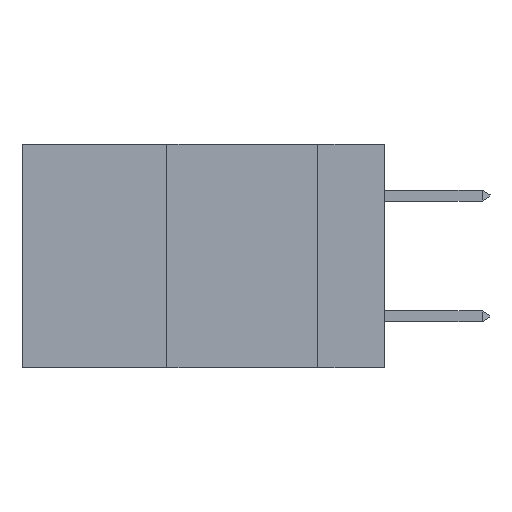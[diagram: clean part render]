
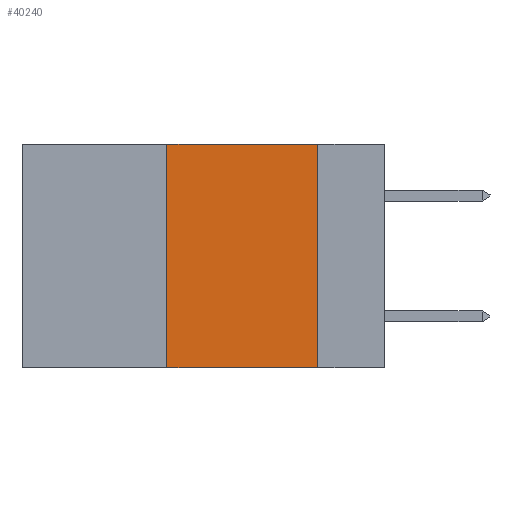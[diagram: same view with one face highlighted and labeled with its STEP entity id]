
A CAD part, left-side view. The second image highlights one B-rep face of the part: STEP entity #40240.
In plain terms, the highlighted planar face has unit normal (-1, 0, 0).
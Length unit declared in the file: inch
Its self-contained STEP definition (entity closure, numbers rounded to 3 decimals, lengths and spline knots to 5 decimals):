
#929 = ORIENTED_EDGE ( 'NONE', *, *, #5429, .F. ) ;
#1715 = EDGE_CURVE ( 'NONE', #12035, #21462, #6893, .T. ) ;
#3799 = EDGE_LOOP ( 'NONE', ( #34235, #929, #30541, #20647 ) ) ;
#4870 = FACE_OUTER_BOUND ( 'NONE', #3799, .T. ) ;
#5429 = EDGE_CURVE ( 'NONE', #21462, #37367, #34326, .T. ) ;
#5641 = EDGE_CURVE ( 'NONE', #12035, #15205, #41756, .T. ) ;
#5966 = CARTESIAN_POINT ( 'NONE',  ( 0., 0.11, 0. ) ) ;
#6170 = CARTESIAN_POINT ( 'NONE',  ( 0., 0.6, -0.37 ) ) ;
#6893 = LINE ( 'NONE', #16922, #13114 ) ;
#11498 = DIRECTION ( 'NONE',  ( 0., 0., -1. ) ) ;
#12035 = VERTEX_POINT ( 'NONE', #40490 ) ;
#12129 = EDGE_CURVE ( 'NONE', #37367, #15205, #12585, .T. ) ;
#12585 = LINE ( 'NONE', #5966, #29763 ) ;
#13114 = VECTOR ( 'NONE', #32696, 39.37008 ) ;
#15205 = VERTEX_POINT ( 'NONE', #28872 ) ;
#16389 = CARTESIAN_POINT ( 'NONE',  ( 0., 0.36, 0. ) ) ;
#16922 = CARTESIAN_POINT ( 'NONE',  ( 0., 0.36, 0. ) ) ;
#20647 = ORIENTED_EDGE ( 'NONE', *, *, #5641, .T. ) ;
#21462 = VERTEX_POINT ( 'NONE', #16389 ) ;
#21908 = AXIS2_PLACEMENT_3D ( 'NONE', #31096, #28131, #11498 ) ;
#21956 = DIRECTION ( 'NONE',  ( 0., -1., 0. ) ) ;
#22389 = VECTOR ( 'NONE', #21956, 39.37008 ) ;
#27395 = CARTESIAN_POINT ( 'NONE',  ( 0., 0.11, 0. ) ) ;
#27505 = DIRECTION ( 'NONE',  ( 0., -1., 0. ) ) ;
#28131 = DIRECTION ( 'NONE',  ( 1., 0., 0. ) ) ;
#28872 = CARTESIAN_POINT ( 'NONE',  ( 0., 0.11, -0.37 ) ) ;
#29763 = VECTOR ( 'NONE', #31982, 39.37008 ) ;
#29866 = VECTOR ( 'NONE', #27505, 39.37008 ) ;
#30541 = ORIENTED_EDGE ( 'NONE', *, *, #1715, .F. ) ;
#31096 = CARTESIAN_POINT ( 'NONE',  ( 0., 0.6, 0. ) ) ;
#31982 = DIRECTION ( 'NONE',  ( 0., 0., -1. ) ) ;
#32696 = DIRECTION ( 'NONE',  ( 0., 0., 1. ) ) ;
#34235 = ORIENTED_EDGE ( 'NONE', *, *, #12129, .F. ) ;
#34326 = LINE ( 'NONE', #37728, #29866 ) ;
#37367 = VERTEX_POINT ( 'NONE', #27395 ) ;
#37728 = CARTESIAN_POINT ( 'NONE',  ( 0., 0.6, 0. ) ) ;
#37918 = PLANE ( 'NONE',  #21908 ) ;
#40240 = ADVANCED_FACE ( 'NONE', ( #4870 ), #37918, .F. ) ;
#40490 = CARTESIAN_POINT ( 'NONE',  ( 0., 0.36, -0.37 ) ) ;
#41756 = LINE ( 'NONE', #6170, #22389 ) ;
